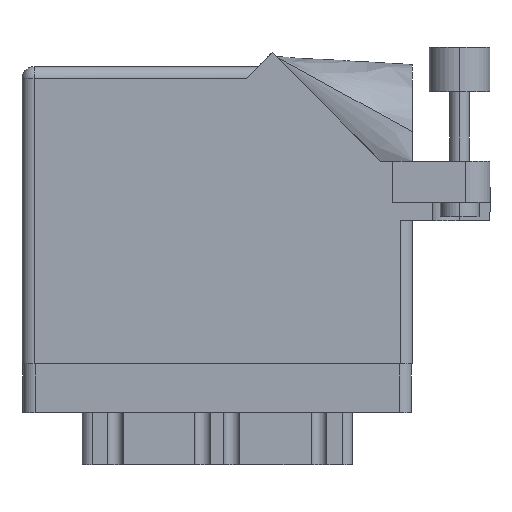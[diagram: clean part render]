
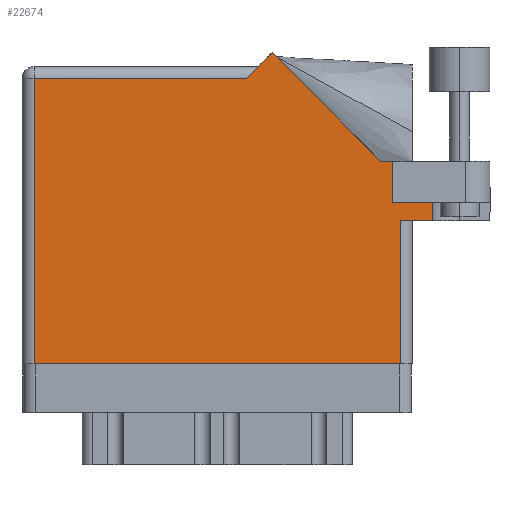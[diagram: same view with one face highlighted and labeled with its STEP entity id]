
A CAD part, front view. The second image highlights one B-rep face of the part: STEP entity #22674.
In plain terms, the highlighted face is planar.
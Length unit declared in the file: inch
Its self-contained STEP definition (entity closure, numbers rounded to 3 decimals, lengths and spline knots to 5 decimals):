
#589 = EDGE_CURVE ( 'NONE', #25609, #12780, #18010, .T. ) ;
#1332 = CARTESIAN_POINT ( 'NONE',  ( 2.41, 1.044, 0. ) ) ;
#2001 = CARTESIAN_POINT ( 'NONE',  ( 0., 1.468, 0. ) ) ;
#2296 = VERTEX_POINT ( 'NONE', #17780 ) ;
#2553 = EDGE_CURVE ( 'NONE', #2296, #9430, #28044, .T. ) ;
#2610 = VECTOR ( 'NONE', #5199, 39.37008 ) ;
#3041 = LINE ( 'NONE', #14740, #14458 ) ;
#3435 = AXIS2_PLACEMENT_3D ( 'NONE', #30605, #36899, #21508 ) ;
#4239 = DIRECTION ( 'NONE',  ( 0., 1., 0. ) ) ;
#4315 = CARTESIAN_POINT ( 'NONE',  ( 2.01, 0.737, 0. ) ) ;
#4532 = VECTOR ( 'NONE', #4239, 39.37008 ) ;
#4828 = CARTESIAN_POINT ( 'NONE',  ( 1.948, 0.737, 0. ) ) ;
#5199 = DIRECTION ( 'NONE',  ( 0., 1., 0. ) ) ;
#5597 = EDGE_LOOP ( 'NONE', ( #15486, #38975, #24232, #11372, #32908, #23090, #32512, #20068, #24690, #18298, #27820 ) ) ;
#5937 = DIRECTION ( 'NONE',  ( -1., 0., 0. ) ) ;
#6117 = CARTESIAN_POINT ( 'NONE',  ( 2.1115, 0.737, 0. ) ) ;
#7511 = EDGE_CURVE ( 'NONE', #14631, #8952, #3041, .T. ) ;
#8408 = DIRECTION ( 'NONE',  ( -0.707, 0.707, 0. ) ) ;
#8952 = VERTEX_POINT ( 'NONE', #6117 ) ;
#9056 = VERTEX_POINT ( 'NONE', #18185 ) ;
#9302 = LINE ( 'NONE', #27528, #12940 ) ;
#9430 = VERTEX_POINT ( 'NONE', #36124 ) ;
#9644 = VERTEX_POINT ( 'NONE', #30985 ) ;
#9815 = FACE_OUTER_BOUND ( 'NONE', #5597, .T. ) ;
#10992 = EDGE_CURVE ( 'NONE', #9430, #23711, #18827, .T. ) ;
#11337 = CARTESIAN_POINT ( 'NONE',  ( 1.155, 1.468, 0. ) ) ;
#11372 = ORIENTED_EDGE ( 'NONE', *, *, #7511, .F. ) ;
#12041 = VECTOR ( 'NONE', #8408, 39.37008 ) ;
#12102 = DIRECTION ( 'NONE',  ( 1., 0., 0. ) ) ;
#12780 = VERTEX_POINT ( 'NONE', #36603 ) ;
#12940 = VECTOR ( 'NONE', #18626, 39.37008 ) ;
#13116 = CARTESIAN_POINT ( 'NONE',  ( 2.1115, 0.831, 0. ) ) ;
#14458 = VECTOR ( 'NONE', #23446, 39.37008 ) ;
#14631 = VERTEX_POINT ( 'NONE', #13116 ) ;
#14740 = CARTESIAN_POINT ( 'NONE',  ( 2.1115, 1.16177, 0. ) ) ;
#14884 = LINE ( 'NONE', #21017, #25366 ) ;
#15270 = CARTESIAN_POINT ( 'NONE',  ( 0.062, 0., 0. ) ) ;
#15486 = ORIENTED_EDGE ( 'NONE', *, *, #17813, .T. ) ;
#16156 = EDGE_CURVE ( 'NONE', #23711, #25609, #9302, .T. ) ;
#16823 = VECTOR ( 'NONE', #37489, 39.37008 ) ;
#16910 = VECTOR ( 'NONE', #22516, 39.37008 ) ;
#17039 = DIRECTION ( 'NONE',  ( 1., 0., 0. ) ) ;
#17780 = CARTESIAN_POINT ( 'NONE',  ( 1.91, 1.044, 0. ) ) ;
#17813 = EDGE_CURVE ( 'NONE', #38160, #9644, #26721, .T. ) ;
#18010 = LINE ( 'NONE', #2001, #19877 ) ;
#18185 = CARTESIAN_POINT ( 'NONE',  ( 1.948, 0.737, 0. ) ) ;
#18298 = ORIENTED_EDGE ( 'NONE', *, *, #589, .T. ) ;
#18626 = DIRECTION ( 'NONE',  ( -0.707, -0.707, 0. ) ) ;
#18664 = CARTESIAN_POINT ( 'NONE',  ( 1.91, 0.831, 0. ) ) ;
#18827 = LINE ( 'NONE', #36398, #12041 ) ;
#18867 = VERTEX_POINT ( 'NONE', #18664 ) ;
#19137 = DIRECTION ( 'NONE',  ( 0., -1., 0. ) ) ;
#19521 = LINE ( 'NONE', #34524, #25991 ) ;
#19672 = LINE ( 'NONE', #4828, #4532 ) ;
#19877 = VECTOR ( 'NONE', #5937, 39.37008 ) ;
#20068 = ORIENTED_EDGE ( 'NONE', *, *, #10992, .T. ) ;
#20303 = CARTESIAN_POINT ( 'NONE',  ( 1.28771, 1.60071, 0. ) ) ;
#21017 = CARTESIAN_POINT ( 'NONE',  ( 1.91, 0.831, 0. ) ) ;
#21508 = DIRECTION ( 'NONE',  ( -1., 0., 0. ) ) ;
#22516 = DIRECTION ( 'NONE',  ( 1., 0., 0. ) ) ;
#22674 = ADVANCED_FACE ( 'NONE', ( #9815 ), #33933, .F. ) ;
#23090 = ORIENTED_EDGE ( 'NONE', *, *, #38129, .T. ) ;
#23446 = DIRECTION ( 'NONE',  ( 0., -1., 0. ) ) ;
#23558 = CARTESIAN_POINT ( 'NONE',  ( 0., 0., 0. ) ) ;
#23711 = VERTEX_POINT ( 'NONE', #20303 ) ;
#24232 = ORIENTED_EDGE ( 'NONE', *, *, #34832, .T. ) ;
#24690 = ORIENTED_EDGE ( 'NONE', *, *, #16156, .T. ) ;
#24894 = EDGE_CURVE ( 'NONE', #12780, #38160, #19521, .T. ) ;
#25366 = VECTOR ( 'NONE', #12102, 39.37008 ) ;
#25609 = VERTEX_POINT ( 'NONE', #11337 ) ;
#25991 = VECTOR ( 'NONE', #19137, 39.37008 ) ;
#26721 = LINE ( 'NONE', #23558, #27953 ) ;
#27528 = CARTESIAN_POINT ( 'NONE',  ( 1.217, 1.53, 0. ) ) ;
#27820 = ORIENTED_EDGE ( 'NONE', *, *, #24894, .T. ) ;
#27892 = EDGE_CURVE ( 'NONE', #18867, #14631, #14884, .T. ) ;
#27953 = VECTOR ( 'NONE', #17039, 39.37008 ) ;
#28044 = LINE ( 'NONE', #1332, #16823 ) ;
#28254 = LINE ( 'NONE', #4315, #16910 ) ;
#29515 = CARTESIAN_POINT ( 'NONE',  ( 1.91, 0.831, 0. ) ) ;
#30605 = CARTESIAN_POINT ( 'NONE',  ( 0., 1.53, 0. ) ) ;
#30781 = EDGE_CURVE ( 'NONE', #9644, #9056, #19672, .T. ) ;
#30985 = CARTESIAN_POINT ( 'NONE',  ( 1.948, 0., 0. ) ) ;
#32282 = LINE ( 'NONE', #29515, #2610 ) ;
#32512 = ORIENTED_EDGE ( 'NONE', *, *, #2553, .T. ) ;
#32908 = ORIENTED_EDGE ( 'NONE', *, *, #27892, .F. ) ;
#33933 = PLANE ( 'NONE',  #3435 ) ;
#34524 = CARTESIAN_POINT ( 'NONE',  ( 0.062, 0., 0. ) ) ;
#34832 = EDGE_CURVE ( 'NONE', #9056, #8952, #28254, .T. ) ;
#36124 = CARTESIAN_POINT ( 'NONE',  ( 1.84442, 1.044, 0. ) ) ;
#36398 = CARTESIAN_POINT ( 'NONE',  ( 1.84442, 1.044, 0. ) ) ;
#36603 = CARTESIAN_POINT ( 'NONE',  ( 0.062, 1.468, 0. ) ) ;
#36899 = DIRECTION ( 'NONE',  ( 0., 0., -1. ) ) ;
#37489 = DIRECTION ( 'NONE',  ( -1., 0., 0. ) ) ;
#38129 = EDGE_CURVE ( 'NONE', #18867, #2296, #32282, .T. ) ;
#38160 = VERTEX_POINT ( 'NONE', #15270 ) ;
#38975 = ORIENTED_EDGE ( 'NONE', *, *, #30781, .T. ) ;
